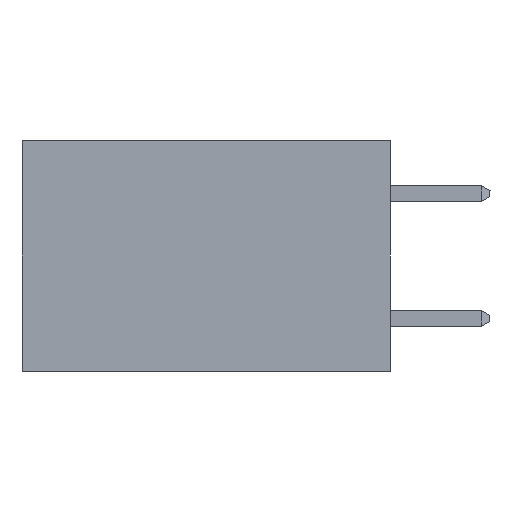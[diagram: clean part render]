
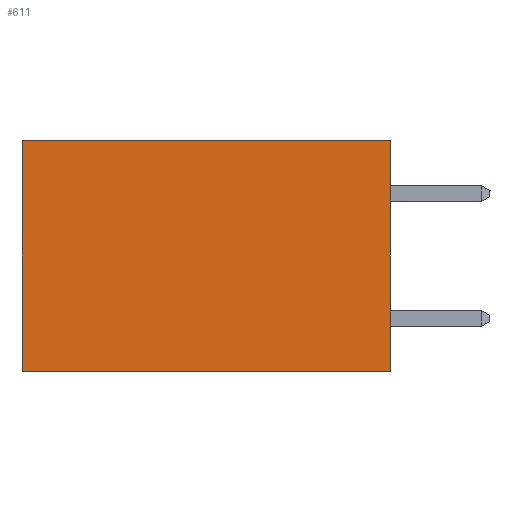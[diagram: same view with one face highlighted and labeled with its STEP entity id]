
A CAD part, left-side view. The second image highlights one B-rep face of the part: STEP entity #611.
In plain terms, the highlighted planar face has unit normal (-1, 0, 0).
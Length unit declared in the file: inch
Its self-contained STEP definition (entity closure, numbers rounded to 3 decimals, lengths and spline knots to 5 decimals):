
#454 = PLANE ( 'NONE',  #7232 ) ;
#611 = ADVANCED_FACE ( 'NONE', ( #14737 ), #454, .F. ) ;
#813 = ORIENTED_EDGE ( 'NONE', *, *, #10935, .T. ) ;
#1520 = EDGE_CURVE ( 'NONE', #5272, #12925, #3497, .T. ) ;
#1784 = CARTESIAN_POINT ( 'NONE',  ( 0.277, 0., 0. ) ) ;
#3497 = LINE ( 'NONE', #1784, #10530 ) ;
#3617 = VECTOR ( 'NONE', #15539, 39.37008 ) ;
#3951 = EDGE_CURVE ( 'NONE', #13521, #5871, #8449, .T. ) ;
#5272 = VERTEX_POINT ( 'NONE', #8427 ) ;
#5705 = CARTESIAN_POINT ( 'NONE',  ( 0.277, 0.59, -0.37 ) ) ;
#5871 = VERTEX_POINT ( 'NONE', #17885 ) ;
#6161 = EDGE_CURVE ( 'NONE', #5272, #13521, #17078, .T. ) ;
#6462 = ORIENTED_EDGE ( 'NONE', *, *, #1520, .T. ) ;
#6877 = LINE ( 'NONE', #5705, #3617 ) ;
#7232 = AXIS2_PLACEMENT_3D ( 'NONE', #12059, #9366, #14801 ) ;
#8427 = CARTESIAN_POINT ( 'NONE',  ( 0.277, 0., 0. ) ) ;
#8449 = LINE ( 'NONE', #14654, #12181 ) ;
#8570 = CARTESIAN_POINT ( 'NONE',  ( 0.277, 0., -0.37 ) ) ;
#8592 = CARTESIAN_POINT ( 'NONE',  ( 0.277, 0.59, 0. ) ) ;
#8808 = DIRECTION ( 'NONE',  ( 0., 0., -1. ) ) ;
#9366 = DIRECTION ( 'NONE',  ( 1., 0., 0. ) ) ;
#10055 = EDGE_LOOP ( 'NONE', ( #813, #10931, #15913, #6462 ) ) ;
#10530 = VECTOR ( 'NONE', #14689, 39.37008 ) ;
#10931 = ORIENTED_EDGE ( 'NONE', *, *, #3951, .F. ) ;
#10935 = EDGE_CURVE ( 'NONE', #12925, #5871, #6877, .T. ) ;
#12059 = CARTESIAN_POINT ( 'NONE',  ( 0.277, 0., -0.37 ) ) ;
#12181 = VECTOR ( 'NONE', #14539, 39.37008 ) ;
#12925 = VERTEX_POINT ( 'NONE', #8592 ) ;
#13521 = VERTEX_POINT ( 'NONE', #15382 ) ;
#14539 = DIRECTION ( 'NONE',  ( 0., 1., 0. ) ) ;
#14654 = CARTESIAN_POINT ( 'NONE',  ( 0.277, 0., -0.37 ) ) ;
#14689 = DIRECTION ( 'NONE',  ( 0., 1., 0. ) ) ;
#14737 = FACE_OUTER_BOUND ( 'NONE', #10055, .T. ) ;
#14801 = DIRECTION ( 'NONE',  ( 0., 0., -1. ) ) ;
#15382 = CARTESIAN_POINT ( 'NONE',  ( 0.277, 0., -0.37 ) ) ;
#15539 = DIRECTION ( 'NONE',  ( 0., 0., -1. ) ) ;
#15913 = ORIENTED_EDGE ( 'NONE', *, *, #6161, .F. ) ;
#16632 = VECTOR ( 'NONE', #8808, 39.37008 ) ;
#17078 = LINE ( 'NONE', #8570, #16632 ) ;
#17885 = CARTESIAN_POINT ( 'NONE',  ( 0.277, 0.59, -0.37 ) ) ;
